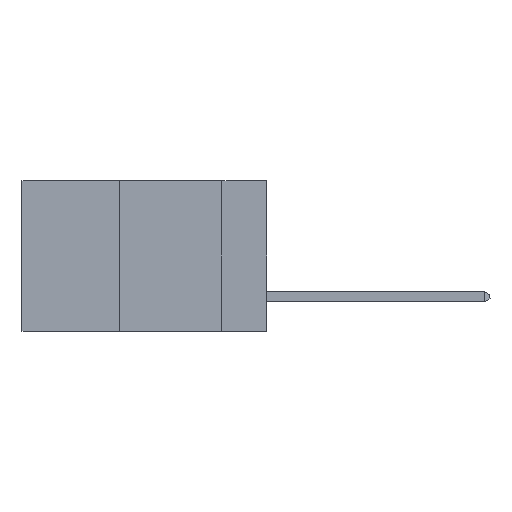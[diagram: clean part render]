
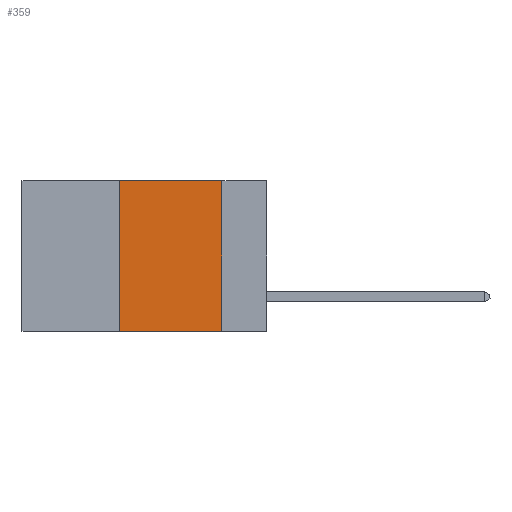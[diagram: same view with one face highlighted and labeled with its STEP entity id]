
A CAD part, left-side view. The second image highlights one B-rep face of the part: STEP entity #359.
In plain terms, the highlighted planar face has unit normal (-1, 0, 0).
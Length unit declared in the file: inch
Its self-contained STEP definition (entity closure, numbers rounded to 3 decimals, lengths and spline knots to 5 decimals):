
#359 = ADVANCED_FACE ( 'NONE', ( #10343 ), #11840, .F. ) ;
#1463 = CARTESIAN_POINT ( 'NONE',  ( 0., 0.11, 0. ) ) ;
#1580 = CARTESIAN_POINT ( 'NONE',  ( 0., 0.6, 0. ) ) ;
#1625 = VERTEX_POINT ( 'NONE', #6127 ) ;
#1869 = VERTEX_POINT ( 'NONE', #5447 ) ;
#1924 = VECTOR ( 'NONE', #3498, 39.37008 ) ;
#2084 = CARTESIAN_POINT ( 'NONE',  ( 0., 0.11, 0. ) ) ;
#2325 = VERTEX_POINT ( 'NONE', #9692 ) ;
#2442 = DIRECTION ( 'NONE',  ( 0., 0., -1. ) ) ;
#2542 = LINE ( 'NONE', #10278, #1924 ) ;
#3402 = AXIS2_PLACEMENT_3D ( 'NONE', #1580, #11109, #2442 ) ;
#3465 = VECTOR ( 'NONE', #12213, 39.37008 ) ;
#3498 = DIRECTION ( 'NONE',  ( 0., 0., 1. ) ) ;
#4589 = VECTOR ( 'NONE', #11767, 39.37008 ) ;
#4793 = EDGE_CURVE ( 'NONE', #9844, #1869, #4907, .T. ) ;
#4907 = LINE ( 'NONE', #2084, #4589 ) ;
#5050 = EDGE_CURVE ( 'NONE', #2325, #1625, #2542, .T. ) ;
#5447 = CARTESIAN_POINT ( 'NONE',  ( 0., 0.11, -0.37 ) ) ;
#5631 = CARTESIAN_POINT ( 'NONE',  ( 0., 0.6, 0. ) ) ;
#5797 = CARTESIAN_POINT ( 'NONE',  ( 0., 0.6, -0.37 ) ) ;
#6127 = CARTESIAN_POINT ( 'NONE',  ( 0., 0.36, 0. ) ) ;
#6265 = EDGE_CURVE ( 'NONE', #1625, #9844, #10594, .T. ) ;
#6388 = EDGE_CURVE ( 'NONE', #2325, #1869, #7460, .T. ) ;
#7360 = ORIENTED_EDGE ( 'NONE', *, *, #6265, .F. ) ;
#7388 = EDGE_LOOP ( 'NONE', ( #8215, #7360, #8035, #7495 ) ) ;
#7460 = LINE ( 'NONE', #5797, #9121 ) ;
#7495 = ORIENTED_EDGE ( 'NONE', *, *, #6388, .T. ) ;
#8035 = ORIENTED_EDGE ( 'NONE', *, *, #5050, .F. ) ;
#8215 = ORIENTED_EDGE ( 'NONE', *, *, #4793, .F. ) ;
#9121 = VECTOR ( 'NONE', #11436, 39.37008 ) ;
#9692 = CARTESIAN_POINT ( 'NONE',  ( 0., 0.36, -0.37 ) ) ;
#9844 = VERTEX_POINT ( 'NONE', #1463 ) ;
#10278 = CARTESIAN_POINT ( 'NONE',  ( 0., 0.36, 0. ) ) ;
#10343 = FACE_OUTER_BOUND ( 'NONE', #7388, .T. ) ;
#10594 = LINE ( 'NONE', #5631, #3465 ) ;
#11109 = DIRECTION ( 'NONE',  ( 1., 0., 0. ) ) ;
#11436 = DIRECTION ( 'NONE',  ( 0., -1., 0. ) ) ;
#11767 = DIRECTION ( 'NONE',  ( 0., 0., -1. ) ) ;
#11840 = PLANE ( 'NONE',  #3402 ) ;
#12213 = DIRECTION ( 'NONE',  ( 0., -1., 0. ) ) ;
